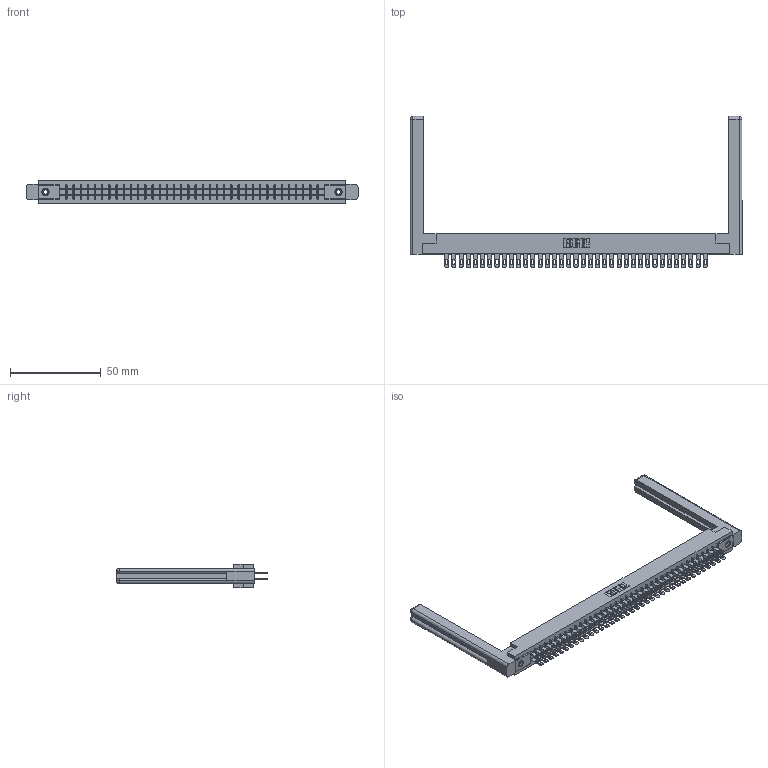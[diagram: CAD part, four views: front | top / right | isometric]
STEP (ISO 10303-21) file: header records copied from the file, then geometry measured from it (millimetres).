
FILE_DESCRIPTION (( 'STEP AP203' ), '1' );
FILE_NAME ('305-074-500-558.STEP', '2019-09-10T06:48:42', ( '' ), ( '' ), 'SwSTEP 2.0', 'SolidWorks 2016', '' );
FILE_SCHEMA (( 'CONFIG_CONTROL_DESIGN' ));
Length unit declared in the file: inch
Products named in the file (5): 345-250-001_345-250-001-102; 307-220-058; 305-290-001_500; 305-074-500-558; 305 Part_.156 Dia
Assembly tree (79 placements, depth 2):
  305-074-500-558
    305 Part_.156 Dia
    305-290-001_500  x74
    345-250-001_345-250-001-102  x2
    307-220-058  x2
Bounding box: 183.24 x 83.49 x 12.7 mm (x, y, z)
Volume: 25959.5 mm3; surface area: 30933.4 mm2
Topology: 79 solids, 79 shells, 3958 faces, 11289 edges, 7314 vertices
Faces by surface type: plane 2224, cylinder 1562, sphere 148, cone 12, torus 12
Entity records: 43325 total; most frequent: CARTESIAN_POINT 7184, ORIENTED_EDGE 7072, DIRECTION 6918, EDGE_CURVE 3536, VECTOR 2842, LINE 2842, VERTEX_POINT 2250, AXIS2_PLACEMENT_3D 2038
